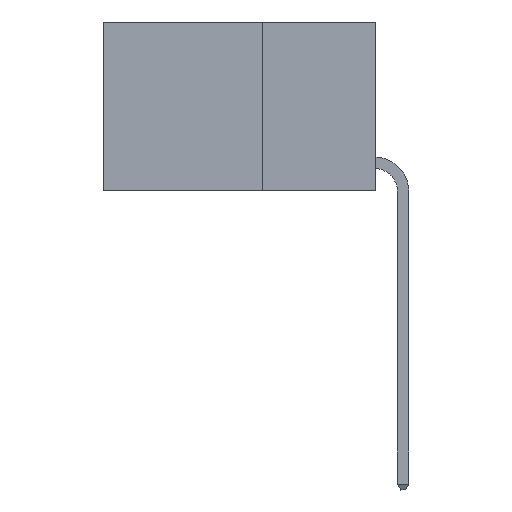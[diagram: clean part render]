
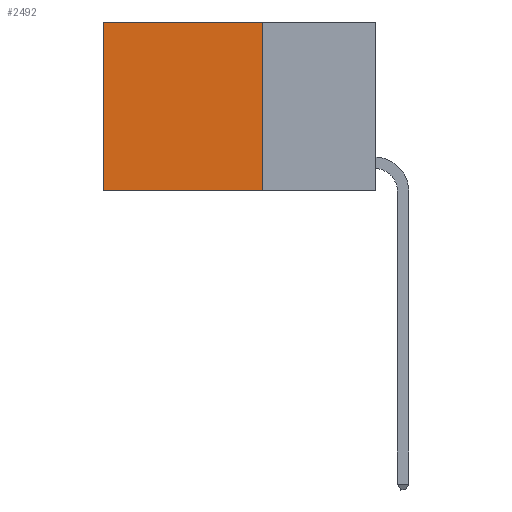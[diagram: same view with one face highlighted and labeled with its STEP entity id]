
A CAD part, left-side view. The second image highlights one B-rep face of the part: STEP entity #2492.
In plain terms, the highlighted planar face has unit normal (-1, 0, 0).
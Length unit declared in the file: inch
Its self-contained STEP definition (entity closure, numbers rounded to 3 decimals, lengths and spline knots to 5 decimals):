
#72 = DIRECTION ( 'NONE',  ( 1., 0., 0. ) ) ;
#791 = DIRECTION ( 'NONE',  ( 0., 1., 0. ) ) ;
#1172 = DIRECTION ( 'NONE',  ( 0., 0., -1. ) ) ;
#1342 = DIRECTION ( 'NONE',  ( 0., 0., -1. ) ) ;
#1953 = VERTEX_POINT ( 'NONE', #9424 ) ;
#2060 = CARTESIAN_POINT ( 'NONE',  ( 0.2625, 0.25, 0. ) ) ;
#2199 = VECTOR ( 'NONE', #4035, 39.37008 ) ;
#2492 = ADVANCED_FACE ( 'NONE', ( #10621 ), #5820, .F. ) ;
#2493 = VERTEX_POINT ( 'NONE', #11059 ) ;
#3079 = LINE ( 'NONE', #5963, #6985 ) ;
#3200 = CARTESIAN_POINT ( 'NONE',  ( 0.2625, 0.6, -0.37 ) ) ;
#3367 = EDGE_CURVE ( 'NONE', #1953, #7794, #3079, .T. ) ;
#4035 = DIRECTION ( 'NONE',  ( 0., 0., -1. ) ) ;
#4568 = EDGE_CURVE ( 'NONE', #2493, #1953, #12204, .T. ) ;
#5062 = DIRECTION ( 'NONE',  ( 0., 1., 0. ) ) ;
#5307 = AXIS2_PLACEMENT_3D ( 'NONE', #9684, #72, #1342 ) ;
#5318 = LINE ( 'NONE', #10169, #10919 ) ;
#5480 = EDGE_CURVE ( 'NONE', #2493, #11738, #10727, .T. ) ;
#5820 = PLANE ( 'NONE',  #5307 ) ;
#5963 = CARTESIAN_POINT ( 'NONE',  ( 0.2625, 0.6, 0. ) ) ;
#6413 = VECTOR ( 'NONE', #791, 39.37008 ) ;
#6985 = VECTOR ( 'NONE', #1172, 39.37008 ) ;
#7434 = CARTESIAN_POINT ( 'NONE',  ( 0.2625, 0.25, 0. ) ) ;
#7580 = CARTESIAN_POINT ( 'NONE',  ( 0.2625, 0.25, -0.37 ) ) ;
#7794 = VERTEX_POINT ( 'NONE', #3200 ) ;
#7825 = EDGE_CURVE ( 'NONE', #11738, #7794, #5318, .T. ) ;
#7976 = ORIENTED_EDGE ( 'NONE', *, *, #3367, .T. ) ;
#8668 = EDGE_LOOP ( 'NONE', ( #7976, #9665, #10215, #9235 ) ) ;
#9235 = ORIENTED_EDGE ( 'NONE', *, *, #4568, .T. ) ;
#9424 = CARTESIAN_POINT ( 'NONE',  ( 0.2625, 0.6, 0. ) ) ;
#9665 = ORIENTED_EDGE ( 'NONE', *, *, #7825, .F. ) ;
#9684 = CARTESIAN_POINT ( 'NONE',  ( 0.2625, 0.25, 0. ) ) ;
#10169 = CARTESIAN_POINT ( 'NONE',  ( 0.2625, 0.25, -0.37 ) ) ;
#10215 = ORIENTED_EDGE ( 'NONE', *, *, #5480, .F. ) ;
#10621 = FACE_OUTER_BOUND ( 'NONE', #8668, .T. ) ;
#10727 = LINE ( 'NONE', #2060, #2199 ) ;
#10919 = VECTOR ( 'NONE', #5062, 39.37008 ) ;
#11059 = CARTESIAN_POINT ( 'NONE',  ( 0.2625, 0.25, 0. ) ) ;
#11738 = VERTEX_POINT ( 'NONE', #7580 ) ;
#12204 = LINE ( 'NONE', #7434, #6413 ) ;
